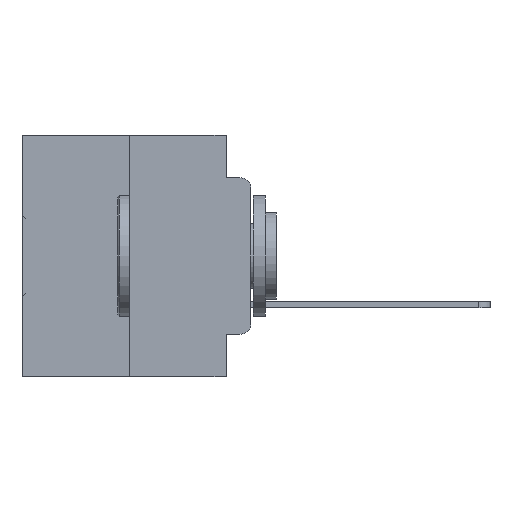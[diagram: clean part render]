
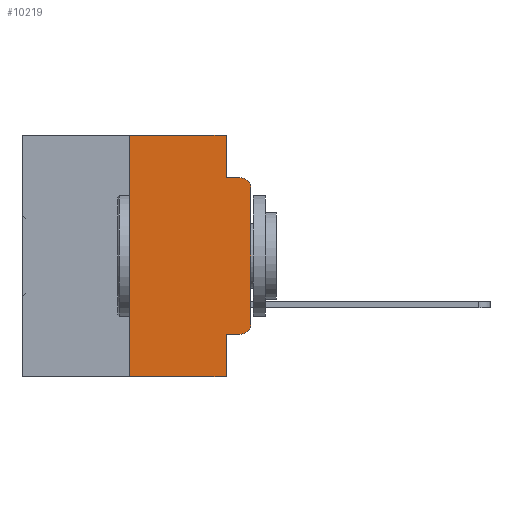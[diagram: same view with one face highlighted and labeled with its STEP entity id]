
A CAD part, left-side view. The second image highlights one B-rep face of the part: STEP entity #10219.
In plain terms, the highlighted planar face has unit normal (-1, 0, 0).
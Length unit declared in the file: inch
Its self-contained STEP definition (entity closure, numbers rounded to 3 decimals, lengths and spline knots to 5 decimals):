
#122 = CIRCLE ( 'NONE', #12470, 0.02 ) ;
#507 = DIRECTION ( 'NONE',  ( 0., 0., 1. ) ) ;
#1095 = CIRCLE ( 'NONE', #3203, 0.02 ) ;
#1627 = VERTEX_POINT ( 'NONE', #29000 ) ;
#2027 = CARTESIAN_POINT ( 'NONE',  ( 0., 0.051, -0.4115 ) ) ;
#2472 = EDGE_CURVE ( 'NONE', #27178, #1627, #18647, .T. ) ;
#2539 = VERTEX_POINT ( 'NONE', #28672 ) ;
#2706 = VECTOR ( 'NONE', #27776, 39.37008 ) ;
#2757 = ORIENTED_EDGE ( 'NONE', *, *, #18531, .F. ) ;
#3203 = AXIS2_PLACEMENT_3D ( 'NONE', #3248, #22535, #6087 ) ;
#3248 = CARTESIAN_POINT ( 'NONE',  ( 0., 0.02, -0.3915 ) ) ;
#3844 = VECTOR ( 'NONE', #23751, 39.37008 ) ;
#3901 = VERTEX_POINT ( 'NONE', #24818 ) ;
#3958 = DIRECTION ( 'NONE',  ( 0., 0., -1. ) ) ;
#4523 = CARTESIAN_POINT ( 'NONE',  ( 0., 0.473, 0. ) ) ;
#4542 = ORIENTED_EDGE ( 'NONE', *, *, #20653, .F. ) ;
#4704 = VECTOR ( 'NONE', #26370, 39.37008 ) ;
#4725 = LINE ( 'NONE', #4523, #3844 ) ;
#4901 = DIRECTION ( 'NONE',  ( 0., -1., 0. ) ) ;
#6087 = DIRECTION ( 'NONE',  ( 0., 0., -1. ) ) ;
#6957 = VECTOR ( 'NONE', #4901, 39.37008 ) ;
#7412 = EDGE_CURVE ( 'NONE', #25317, #3901, #28814, .T. ) ;
#7433 = EDGE_LOOP ( 'NONE', ( #27762, #15074, #16805, #2757, #25262, #4542, #12028, #27485, #14658, #15531 ) ) ;
#7783 = CARTESIAN_POINT ( 'NONE',  ( 0., 0., -0.1085 ) ) ;
#8058 = EDGE_CURVE ( 'NONE', #24257, #32459, #32353, .T. ) ;
#9815 = CARTESIAN_POINT ( 'NONE',  ( 0., 0.051, 0. ) ) ;
#10219 = ADVANCED_FACE ( 'NONE', ( #12208 ), #23646, .F. ) ;
#10234 = DIRECTION ( 'NONE',  ( 0., 0., -1. ) ) ;
#10262 = LINE ( 'NONE', #25392, #2706 ) ;
#10605 = CARTESIAN_POINT ( 'NONE',  ( 0., 0., 0. ) ) ;
#10797 = CARTESIAN_POINT ( 'NONE',  ( 0., 0.25, 0. ) ) ;
#11771 = LINE ( 'NONE', #23133, #24311 ) ;
#12028 = ORIENTED_EDGE ( 'NONE', *, *, #2472, .T. ) ;
#12208 = FACE_OUTER_BOUND ( 'NONE', #7433, .T. ) ;
#12341 = VECTOR ( 'NONE', #507, 39.37008 ) ;
#12470 = AXIS2_PLACEMENT_3D ( 'NONE', #16192, #33396, #18941 ) ;
#14658 = ORIENTED_EDGE ( 'NONE', *, *, #7412, .T. ) ;
#15074 = ORIENTED_EDGE ( 'NONE', *, *, #25950, .T. ) ;
#15200 = CARTESIAN_POINT ( 'NONE',  ( 0., 0., -0.3915 ) ) ;
#15531 = ORIENTED_EDGE ( 'NONE', *, *, #25014, .T. ) ;
#15601 = VERTEX_POINT ( 'NONE', #30576 ) ;
#16192 = CARTESIAN_POINT ( 'NONE',  ( 0., 0.02, -0.1085 ) ) ;
#16805 = ORIENTED_EDGE ( 'NONE', *, *, #30680, .F. ) ;
#17393 = CARTESIAN_POINT ( 'NONE',  ( 0., 0.25, 0. ) ) ;
#18239 = AXIS2_PLACEMENT_3D ( 'NONE', #28322, #26067, #10234 ) ;
#18531 = EDGE_CURVE ( 'NONE', #15601, #2539, #11771, .T. ) ;
#18647 = LINE ( 'NONE', #25989, #30912 ) ;
#18941 = DIRECTION ( 'NONE',  ( 0., 0., -1. ) ) ;
#20653 = EDGE_CURVE ( 'NONE', #27178, #25804, #25518, .T. ) ;
#21169 = DIRECTION ( 'NONE',  ( 0., -1., 0. ) ) ;
#21902 = EDGE_CURVE ( 'NONE', #25804, #15601, #4725, .T. ) ;
#22535 = DIRECTION ( 'NONE',  ( -1., 0., 0. ) ) ;
#22749 = EDGE_CURVE ( 'NONE', #25317, #1627, #30918, .T. ) ;
#23133 = CARTESIAN_POINT ( 'NONE',  ( 0., 0.051, 0. ) ) ;
#23397 = DIRECTION ( 'NONE',  ( 0., 0., -1. ) ) ;
#23646 = PLANE ( 'NONE',  #18239 ) ;
#23751 = DIRECTION ( 'NONE',  ( 0., -1., 0. ) ) ;
#24257 = VERTEX_POINT ( 'NONE', #15200 ) ;
#24311 = VECTOR ( 'NONE', #3958, 39.37008 ) ;
#24818 = CARTESIAN_POINT ( 'NONE',  ( 0., 0.02, -0.4115 ) ) ;
#25014 = EDGE_CURVE ( 'NONE', #3901, #24257, #1095, .T. ) ;
#25262 = ORIENTED_EDGE ( 'NONE', *, *, #21902, .F. ) ;
#25317 = VERTEX_POINT ( 'NONE', #30240 ) ;
#25392 = CARTESIAN_POINT ( 'NONE',  ( 0., 0.051, -0.0885 ) ) ;
#25518 = LINE ( 'NONE', #17393, #12341 ) ;
#25804 = VERTEX_POINT ( 'NONE', #10797 ) ;
#25950 = EDGE_CURVE ( 'NONE', #32459, #31942, #122, .T. ) ;
#25989 = CARTESIAN_POINT ( 'NONE',  ( 0., 0.473, -0.5 ) ) ;
#26067 = DIRECTION ( 'NONE',  ( 1., 0., 0. ) ) ;
#26370 = DIRECTION ( 'NONE',  ( 0., 0., 1. ) ) ;
#27178 = VERTEX_POINT ( 'NONE', #33756 ) ;
#27485 = ORIENTED_EDGE ( 'NONE', *, *, #22749, .F. ) ;
#27762 = ORIENTED_EDGE ( 'NONE', *, *, #8058, .T. ) ;
#27776 = DIRECTION ( 'NONE',  ( 0., -1., 0. ) ) ;
#28322 = CARTESIAN_POINT ( 'NONE',  ( 0., 0.473, 0. ) ) ;
#28672 = CARTESIAN_POINT ( 'NONE',  ( 0., 0.051, -0.0885 ) ) ;
#28814 = LINE ( 'NONE', #2027, #6957 ) ;
#29000 = CARTESIAN_POINT ( 'NONE',  ( 0., 0.051, -0.5 ) ) ;
#30193 = VECTOR ( 'NONE', #23397, 39.37008 ) ;
#30240 = CARTESIAN_POINT ( 'NONE',  ( 0., 0.051, -0.4115 ) ) ;
#30576 = CARTESIAN_POINT ( 'NONE',  ( 0., 0.051, 0. ) ) ;
#30680 = EDGE_CURVE ( 'NONE', #2539, #31942, #10262, .T. ) ;
#30912 = VECTOR ( 'NONE', #21169, 39.37008 ) ;
#30918 = LINE ( 'NONE', #9815, #30193 ) ;
#31942 = VERTEX_POINT ( 'NONE', #32141 ) ;
#32141 = CARTESIAN_POINT ( 'NONE',  ( 0., 0.02, -0.0885 ) ) ;
#32353 = LINE ( 'NONE', #10605, #4704 ) ;
#32459 = VERTEX_POINT ( 'NONE', #7783 ) ;
#33396 = DIRECTION ( 'NONE',  ( -1., 0., 0. ) ) ;
#33756 = CARTESIAN_POINT ( 'NONE',  ( 0., 0.25, -0.5 ) ) ;
